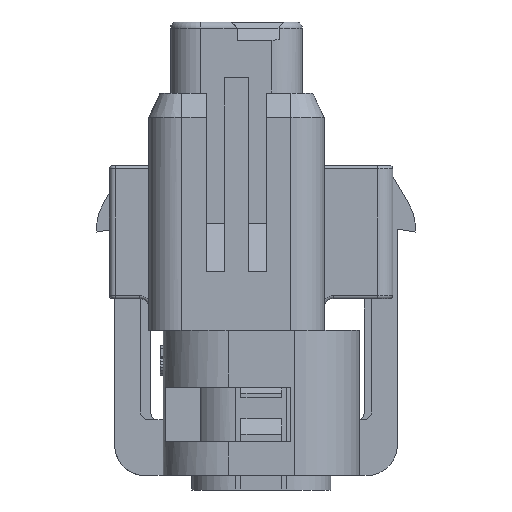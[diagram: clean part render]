
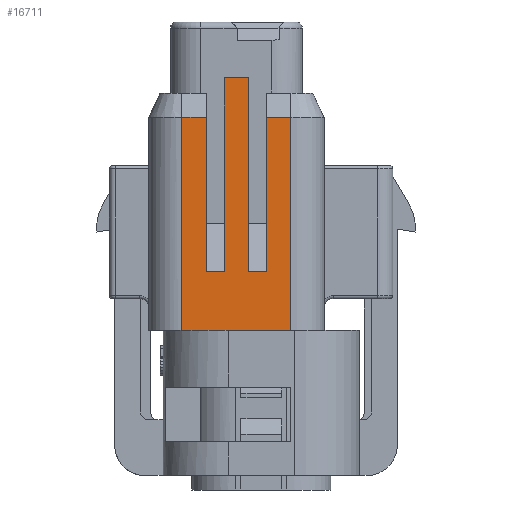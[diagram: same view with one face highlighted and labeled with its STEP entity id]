
A CAD part, left-side view. The second image highlights one B-rep face of the part: STEP entity #16711.
In plain terms, the highlighted planar face has unit normal (-1, 0, 0).
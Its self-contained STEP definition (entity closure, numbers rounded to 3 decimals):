
#441 = EDGE_CURVE ( 'NONE', #10608, #21295, #20550, .T. ) ;
#580 = CARTESIAN_POINT ( 'NONE',  ( 1.1, 5.225, -22.03 ) ) ;
#732 = CARTESIAN_POINT ( 'NONE',  ( 1.1, 8.025, -16.93 ) ) ;
#757 = VERTEX_POINT ( 'NONE', #17937 ) ;
#802 = EDGE_CURVE ( 'NONE', #19873, #4612, #11792, .T. ) ;
#1665 = CARTESIAN_POINT ( 'NONE',  ( 1.1, 8.025, -23.98 ) ) ;
#1708 = ORIENTED_EDGE ( 'NONE', *, *, #802, .T. ) ;
#2025 = DIRECTION ( 'NONE',  ( 0., 0., -1. ) ) ;
#2891 = CARTESIAN_POINT ( 'NONE',  ( 1.1, 5.225, -22.03 ) ) ;
#3523 = LINE ( 'NONE', #12920, #27423 ) ;
#3680 = LINE ( 'NONE', #19801, #27784 ) ;
#3710 = DIRECTION ( 'NONE',  ( 0., 0., 1. ) ) ;
#4612 = VERTEX_POINT ( 'NONE', #21154 ) ;
#5199 = EDGE_CURVE ( 'NONE', #757, #26877, #5880, .T. ) ;
#5349 = LINE ( 'NONE', #23602, #12140 ) ;
#5592 = ORIENTED_EDGE ( 'NONE', *, *, #7606, .T. ) ;
#5880 = LINE ( 'NONE', #6030, #22195 ) ;
#6030 = CARTESIAN_POINT ( 'NONE',  ( 1.1, 6.625, -15.63 ) ) ;
#6284 = DIRECTION ( 'NONE',  ( 0., 0., -1. ) ) ;
#6946 = DIRECTION ( 'NONE',  ( 0., -1., 0. ) ) ;
#7002 = DIRECTION ( 'NONE',  ( 0., 1., 0. ) ) ;
#7567 = CARTESIAN_POINT ( 'NONE',  ( 1.1, 9.125, -23.98 ) ) ;
#7606 = EDGE_CURVE ( 'NONE', #26851, #19873, #19950, .T. ) ;
#8028 = ORIENTED_EDGE ( 'NONE', *, *, #29491, .T. ) ;
#9180 = CARTESIAN_POINT ( 'NONE',  ( 1.1, 5.225, -16.93 ) ) ;
#9664 = DIRECTION ( 'NONE',  ( 0., 1., 0. ) ) ;
#10262 = CARTESIAN_POINT ( 'NONE',  ( 1.1, 5.825, -22.03 ) ) ;
#10273 = CARTESIAN_POINT ( 'NONE',  ( 1.1, 7.225, -16.93 ) ) ;
#10608 = VERTEX_POINT ( 'NONE', #11799 ) ;
#10963 = LINE ( 'NONE', #20088, #18674 ) ;
#11035 = ORIENTED_EDGE ( 'NONE', *, *, #5199, .F. ) ;
#11036 = ORIENTED_EDGE ( 'NONE', *, *, #17766, .F. ) ;
#11041 = EDGE_CURVE ( 'NONE', #23760, #14618, #23592, .T. ) ;
#11792 = LINE ( 'NONE', #25142, #23387 ) ;
#11799 = CARTESIAN_POINT ( 'NONE',  ( 1.1, 5.225, -16.93 ) ) ;
#12140 = VECTOR ( 'NONE', #7002, 1000. ) ;
#12628 = DIRECTION ( 'NONE',  ( 0., 0., 1. ) ) ;
#12920 = CARTESIAN_POINT ( 'NONE',  ( 1.1, 4.425, -16.93 ) ) ;
#13033 = CARTESIAN_POINT ( 'NONE',  ( 1.1, 8.025, -16.93 ) ) ;
#13063 = DIRECTION ( 'NONE',  ( 0., 0., -1. ) ) ;
#14212 = CARTESIAN_POINT ( 'NONE',  ( 1.1, 5.825, -22.03 ) ) ;
#14234 = EDGE_CURVE ( 'NONE', #26851, #18443, #22022, .T. ) ;
#14437 = DIRECTION ( 'NONE',  ( -1., 0., 0. ) ) ;
#14618 = VERTEX_POINT ( 'NONE', #14212 ) ;
#14860 = VERTEX_POINT ( 'NONE', #27520 ) ;
#15132 = DIRECTION ( 'NONE',  ( 0., -1., 0. ) ) ;
#15612 = ORIENTED_EDGE ( 'NONE', *, *, #19949, .T. ) ;
#15834 = ORIENTED_EDGE ( 'NONE', *, *, #17789, .T. ) ;
#16240 = VECTOR ( 'NONE', #3710, 1000. ) ;
#16407 = VECTOR ( 'NONE', #21612, 1000. ) ;
#16528 = FACE_OUTER_BOUND ( 'NONE', #17778, .T. ) ;
#16694 = LINE ( 'NONE', #10262, #16240 ) ;
#16711 = ADVANCED_FACE ( 'NONE', ( #16528 ), #28081, .T. ) ;
#17409 = CARTESIAN_POINT ( 'NONE',  ( 1.1, 8.025, -16.93 ) ) ;
#17766 = EDGE_CURVE ( 'NONE', #21295, #4612, #3523, .T. ) ;
#17778 = EDGE_LOOP ( 'NONE', ( #24848, #18013, #8028, #11035, #15612, #27371, #15834, #19973, #5592, #1708, #11036, #29593 ) ) ;
#17789 = EDGE_CURVE ( 'NONE', #14860, #18443, #3680, .T. ) ;
#17868 = EDGE_CURVE ( 'NONE', #10608, #23760, #10963, .T. ) ;
#17937 = CARTESIAN_POINT ( 'NONE',  ( 1.1, 6.625, -15.63 ) ) ;
#18013 = ORIENTED_EDGE ( 'NONE', *, *, #11041, .T. ) ;
#18443 = VERTEX_POINT ( 'NONE', #10273 ) ;
#18674 = VECTOR ( 'NONE', #2025, 1000. ) ;
#19801 = CARTESIAN_POINT ( 'NONE',  ( 1.1, 7.225, -22.03 ) ) ;
#19873 = VERTEX_POINT ( 'NONE', #1665 ) ;
#19949 = EDGE_CURVE ( 'NONE', #757, #27227, #22439, .T. ) ;
#19950 = LINE ( 'NONE', #17409, #16407 ) ;
#19973 = ORIENTED_EDGE ( 'NONE', *, *, #14234, .F. ) ;
#20088 = CARTESIAN_POINT ( 'NONE',  ( 1.1, 5.225, -16.93 ) ) ;
#20172 = CARTESIAN_POINT ( 'NONE',  ( 1.1, 6.625, -15.63 ) ) ;
#20550 = LINE ( 'NONE', #9180, #24503 ) ;
#20567 = CARTESIAN_POINT ( 'NONE',  ( 1.1, 6.625, -22.03 ) ) ;
#21154 = CARTESIAN_POINT ( 'NONE',  ( 1.1, 4.425, -23.98 ) ) ;
#21295 = VERTEX_POINT ( 'NONE', #27674 ) ;
#21329 = DIRECTION ( 'NONE',  ( 0., -1., 0. ) ) ;
#21612 = DIRECTION ( 'NONE',  ( 0., 0., -1. ) ) ;
#21883 = DIRECTION ( 'NONE',  ( 0., -1., 0. ) ) ;
#22022 = LINE ( 'NONE', #13033, #27054 ) ;
#22195 = VECTOR ( 'NONE', #15132, 1000. ) ;
#22326 = VECTOR ( 'NONE', #6284, 1000. ) ;
#22439 = LINE ( 'NONE', #20172, #22326 ) ;
#22748 = DIRECTION ( 'NONE',  ( 0., -1., 0. ) ) ;
#23142 = CARTESIAN_POINT ( 'NONE',  ( 1.1, 5.825, -15.63 ) ) ;
#23387 = VECTOR ( 'NONE', #22748, 1000. ) ;
#23592 = LINE ( 'NONE', #580, #28258 ) ;
#23602 = CARTESIAN_POINT ( 'NONE',  ( 1.1, 6.625, -22.03 ) ) ;
#23760 = VERTEX_POINT ( 'NONE', #2891 ) ;
#24028 = AXIS2_PLACEMENT_3D ( 'NONE', #7567, #14437, #21329 ) ;
#24503 = VECTOR ( 'NONE', #6946, 1000. ) ;
#24565 = EDGE_CURVE ( 'NONE', #27227, #14860, #5349, .T. ) ;
#24848 = ORIENTED_EDGE ( 'NONE', *, *, #17868, .T. ) ;
#25142 = CARTESIAN_POINT ( 'NONE',  ( 1.1, 8.025, -23.98 ) ) ;
#26851 = VERTEX_POINT ( 'NONE', #732 ) ;
#26877 = VERTEX_POINT ( 'NONE', #23142 ) ;
#27054 = VECTOR ( 'NONE', #21883, 1000. ) ;
#27227 = VERTEX_POINT ( 'NONE', #20567 ) ;
#27371 = ORIENTED_EDGE ( 'NONE', *, *, #24565, .T. ) ;
#27423 = VECTOR ( 'NONE', #13063, 1000. ) ;
#27520 = CARTESIAN_POINT ( 'NONE',  ( 1.1, 7.225, -22.03 ) ) ;
#27674 = CARTESIAN_POINT ( 'NONE',  ( 1.1, 4.425, -16.93 ) ) ;
#27784 = VECTOR ( 'NONE', #12628, 1000. ) ;
#28081 = PLANE ( 'NONE',  #24028 ) ;
#28258 = VECTOR ( 'NONE', #9664, 1000. ) ;
#29491 = EDGE_CURVE ( 'NONE', #14618, #26877, #16694, .T. ) ;
#29593 = ORIENTED_EDGE ( 'NONE', *, *, #441, .F. ) ;
